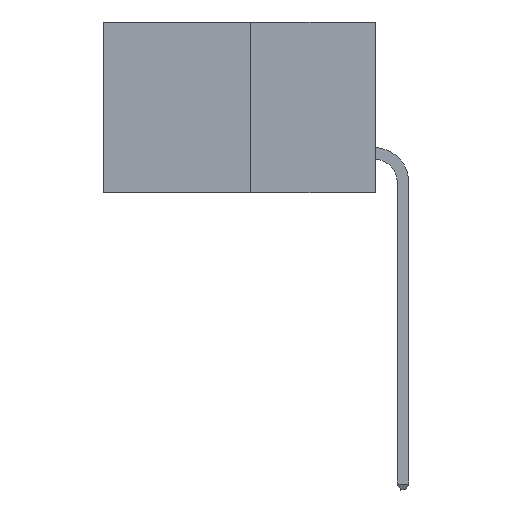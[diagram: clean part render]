
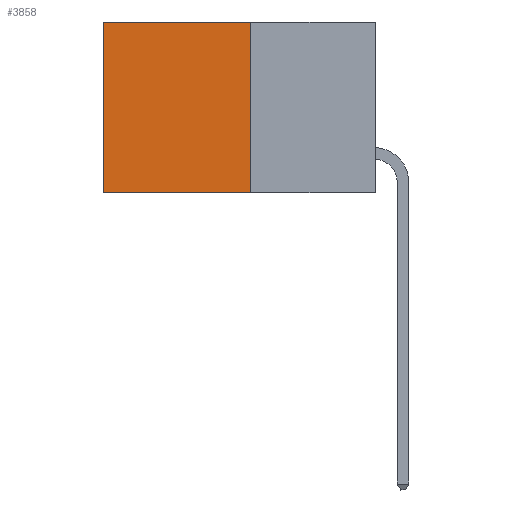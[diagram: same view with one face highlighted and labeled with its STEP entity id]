
A CAD part, left-side view. The second image highlights one B-rep face of the part: STEP entity #3858.
In plain terms, the highlighted planar face has unit normal (-1, 0, 0).
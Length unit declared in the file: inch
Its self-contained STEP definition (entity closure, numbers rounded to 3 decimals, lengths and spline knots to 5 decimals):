
#87 = EDGE_CURVE ( 'NONE', #6889, #1319, #2968, .T. ) ;
#205 = DIRECTION ( 'NONE',  ( 0., 1., 0. ) ) ;
#660 = CARTESIAN_POINT ( 'NONE',  ( 0.277, 0.59, -0.37 ) ) ;
#1319 = VERTEX_POINT ( 'NONE', #10993 ) ;
#1388 = DIRECTION ( 'NONE',  ( 0., 1., 0. ) ) ;
#1438 = CARTESIAN_POINT ( 'NONE',  ( 0.277, 0.27, -0.37 ) ) ;
#1466 = CARTESIAN_POINT ( 'NONE',  ( 0.277, 0.27, -0.37 ) ) ;
#1709 = CARTESIAN_POINT ( 'NONE',  ( 0.277, 0.59, 0. ) ) ;
#1863 = LINE ( 'NONE', #2656, #4174 ) ;
#2181 = ORIENTED_EDGE ( 'NONE', *, *, #9052, .T. ) ;
#2401 = VERTEX_POINT ( 'NONE', #660 ) ;
#2491 = CARTESIAN_POINT ( 'NONE',  ( 0.277, 0.27, 0. ) ) ;
#2656 = CARTESIAN_POINT ( 'NONE',  ( 0.277, 0.59, -0.37 ) ) ;
#2968 = LINE ( 'NONE', #1438, #5256 ) ;
#3080 = CARTESIAN_POINT ( 'NONE',  ( 0.277, 0.27, 0. ) ) ;
#3588 = FACE_OUTER_BOUND ( 'NONE', #11882, .T. ) ;
#3609 = DIRECTION ( 'NONE',  ( 0., 0., -1. ) ) ;
#3851 = DIRECTION ( 'NONE',  ( 1., 0., 0. ) ) ;
#3858 = ADVANCED_FACE ( 'NONE', ( #3588 ), #4687, .F. ) ;
#4141 = CARTESIAN_POINT ( 'NONE',  ( 0.277, 0.27, -0.37 ) ) ;
#4174 = VECTOR ( 'NONE', #12012, 39.37008 ) ;
#4687 = PLANE ( 'NONE',  #7466 ) ;
#5256 = VECTOR ( 'NONE', #6831, 39.37008 ) ;
#5300 = VERTEX_POINT ( 'NONE', #1709 ) ;
#5302 = EDGE_CURVE ( 'NONE', #1319, #2401, #12191, .T. ) ;
#6664 = EDGE_CURVE ( 'NONE', #6889, #5300, #8098, .T. ) ;
#6831 = DIRECTION ( 'NONE',  ( 0., 0., -1. ) ) ;
#6889 = VERTEX_POINT ( 'NONE', #2491 ) ;
#7466 = AXIS2_PLACEMENT_3D ( 'NONE', #4141, #3851, #3609 ) ;
#7541 = ORIENTED_EDGE ( 'NONE', *, *, #6664, .T. ) ;
#8098 = LINE ( 'NONE', #3080, #8386 ) ;
#8386 = VECTOR ( 'NONE', #205, 39.37008 ) ;
#9052 = EDGE_CURVE ( 'NONE', #5300, #2401, #1863, .T. ) ;
#9753 = ORIENTED_EDGE ( 'NONE', *, *, #5302, .F. ) ;
#9763 = VECTOR ( 'NONE', #1388, 39.37008 ) ;
#10993 = CARTESIAN_POINT ( 'NONE',  ( 0.277, 0.27, -0.37 ) ) ;
#11882 = EDGE_LOOP ( 'NONE', ( #2181, #9753, #12180, #7541 ) ) ;
#12012 = DIRECTION ( 'NONE',  ( 0., 0., -1. ) ) ;
#12180 = ORIENTED_EDGE ( 'NONE', *, *, #87, .F. ) ;
#12191 = LINE ( 'NONE', #1466, #9763 ) ;
